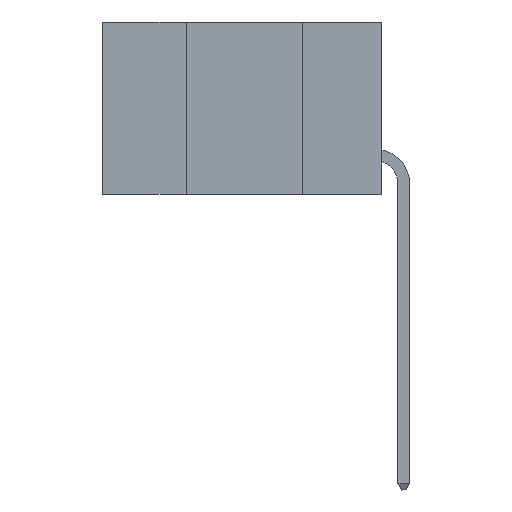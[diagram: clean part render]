
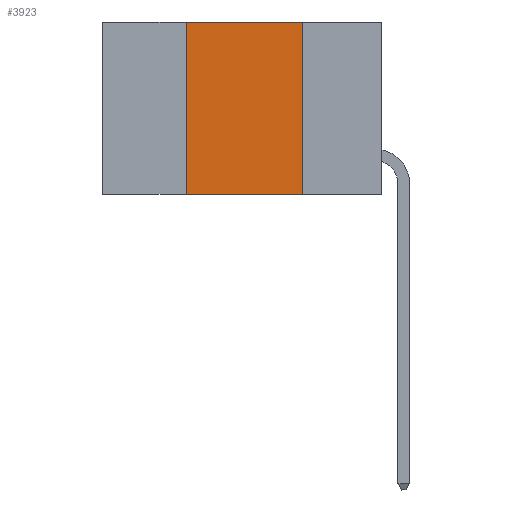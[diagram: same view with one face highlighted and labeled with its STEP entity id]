
A CAD part, left-side view. The second image highlights one B-rep face of the part: STEP entity #3923.
In plain terms, the highlighted planar face has unit normal (-1, 0, 0).
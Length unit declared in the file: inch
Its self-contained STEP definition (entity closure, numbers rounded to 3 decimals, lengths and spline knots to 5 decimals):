
#18 = ORIENTED_EDGE ( 'NONE', *, *, #7673, .T. ) ;
#630 = EDGE_LOOP ( 'NONE', ( #4988, #9325, #1724, #18 ) ) ;
#838 = CARTESIAN_POINT ( 'NONE',  ( 0., 0.42, -0.37 ) ) ;
#927 = DIRECTION ( 'NONE',  ( 0., -1., 0. ) ) ;
#1595 = DIRECTION ( 'NONE',  ( 0., 0., -1. ) ) ;
#1724 = ORIENTED_EDGE ( 'NONE', *, *, #11932, .F. ) ;
#1838 = DIRECTION ( 'NONE',  ( 0., 0., 1. ) ) ;
#2387 = LINE ( 'NONE', #9229, #3818 ) ;
#3066 = LINE ( 'NONE', #8015, #11566 ) ;
#3220 = DIRECTION ( 'NONE',  ( 0., -1., 0. ) ) ;
#3451 = VECTOR ( 'NONE', #11931, 39.37008 ) ;
#3818 = VECTOR ( 'NONE', #3220, 39.37008 ) ;
#3923 = ADVANCED_FACE ( 'NONE', ( #7844 ), #11635, .F. ) ;
#4136 = VERTEX_POINT ( 'NONE', #8898 ) ;
#4988 = ORIENTED_EDGE ( 'NONE', *, *, #8854, .F. ) ;
#5100 = CARTESIAN_POINT ( 'NONE',  ( 0., 0.6, 0. ) ) ;
#6564 = CARTESIAN_POINT ( 'NONE',  ( 0., 0.6, 0. ) ) ;
#7673 = EDGE_CURVE ( 'NONE', #11210, #8828, #2387, .T. ) ;
#7844 = FACE_OUTER_BOUND ( 'NONE', #630, .T. ) ;
#7882 = CARTESIAN_POINT ( 'NONE',  ( 0., 0.17, -0.37 ) ) ;
#8015 = CARTESIAN_POINT ( 'NONE',  ( 0., 0.42, 0. ) ) ;
#8141 = AXIS2_PLACEMENT_3D ( 'NONE', #6564, #8686, #1595 ) ;
#8686 = DIRECTION ( 'NONE',  ( 1., 0., 0. ) ) ;
#8828 = VERTEX_POINT ( 'NONE', #7882 ) ;
#8854 = EDGE_CURVE ( 'NONE', #4136, #8828, #11170, .T. ) ;
#8898 = CARTESIAN_POINT ( 'NONE',  ( 0., 0.17, 0. ) ) ;
#9229 = CARTESIAN_POINT ( 'NONE',  ( 0., 0.6, -0.37 ) ) ;
#9325 = ORIENTED_EDGE ( 'NONE', *, *, #10772, .F. ) ;
#9488 = LINE ( 'NONE', #5100, #10281 ) ;
#9684 = VERTEX_POINT ( 'NONE', #10075 ) ;
#9951 = CARTESIAN_POINT ( 'NONE',  ( 0., 0.17, 0. ) ) ;
#10075 = CARTESIAN_POINT ( 'NONE',  ( 0., 0.42, 0. ) ) ;
#10281 = VECTOR ( 'NONE', #927, 39.37008 ) ;
#10772 = EDGE_CURVE ( 'NONE', #9684, #4136, #9488, .T. ) ;
#11170 = LINE ( 'NONE', #9951, #3451 ) ;
#11210 = VERTEX_POINT ( 'NONE', #838 ) ;
#11566 = VECTOR ( 'NONE', #1838, 39.37008 ) ;
#11635 = PLANE ( 'NONE',  #8141 ) ;
#11931 = DIRECTION ( 'NONE',  ( 0., 0., -1. ) ) ;
#11932 = EDGE_CURVE ( 'NONE', #11210, #9684, #3066, .T. ) ;
